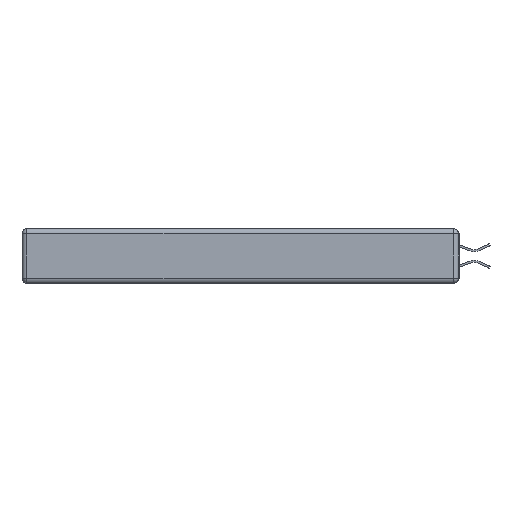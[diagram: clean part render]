
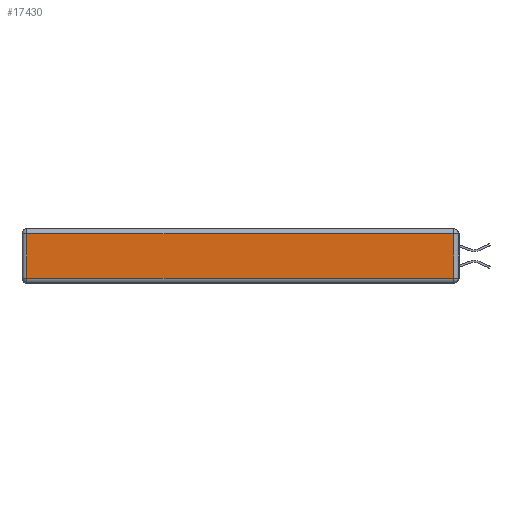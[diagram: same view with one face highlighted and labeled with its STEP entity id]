
A CAD part, left-side view. The second image highlights one B-rep face of the part: STEP entity #17430.
In plain terms, the highlighted planar face has unit normal (-1, 0, 0).
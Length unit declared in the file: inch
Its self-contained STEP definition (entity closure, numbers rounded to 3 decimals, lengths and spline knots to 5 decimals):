
#206 = ORIENTED_EDGE ( 'NONE', *, *, #7470, .T. ) ;
#953 = ORIENTED_EDGE ( 'NONE', *, *, #4564, .T. ) ;
#1438 = LINE ( 'NONE', #15398, #14911 ) ;
#2164 = VECTOR ( 'NONE', #7937, 39.37008 ) ;
#2230 = CARTESIAN_POINT ( 'NONE',  ( 0., 2.75, -0.03 ) ) ;
#3744 = VERTEX_POINT ( 'NONE', #12139 ) ;
#4537 = DIRECTION ( 'NONE',  ( 0., -1., 0. ) ) ;
#4564 = EDGE_CURVE ( 'NONE', #11316, #7080, #1438, .T. ) ;
#4608 = CARTESIAN_POINT ( 'NONE',  ( 0., 0.03, -0.343 ) ) ;
#4664 = DIRECTION ( 'NONE',  ( -1., 0., 0. ) ) ;
#5738 = EDGE_LOOP ( 'NONE', ( #206, #11890, #14962, #953 ) ) ;
#5791 = LINE ( 'NONE', #4608, #2164 ) ;
#6066 = CARTESIAN_POINT ( 'NONE',  ( 0., 0.03, -0.313 ) ) ;
#7080 = VERTEX_POINT ( 'NONE', #13982 ) ;
#7470 = EDGE_CURVE ( 'NONE', #7080, #8627, #12040, .T. ) ;
#7937 = DIRECTION ( 'NONE',  ( 0., 0., 1. ) ) ;
#8220 = VECTOR ( 'NONE', #4537, 39.37008 ) ;
#8518 = VECTOR ( 'NONE', #10351, 39.37008 ) ;
#8627 = VERTEX_POINT ( 'NONE', #6066 ) ;
#8651 = DIRECTION ( 'NONE',  ( 0., 0., -1. ) ) ;
#10269 = CARTESIAN_POINT ( 'NONE',  ( 0., 0., -0.343 ) ) ;
#10351 = DIRECTION ( 'NONE',  ( 0., 1., 0. ) ) ;
#11195 = EDGE_CURVE ( 'NONE', #3744, #11316, #17252, .T. ) ;
#11316 = VERTEX_POINT ( 'NONE', #12196 ) ;
#11890 = ORIENTED_EDGE ( 'NONE', *, *, #17446, .T. ) ;
#12040 = LINE ( 'NONE', #13924, #8220 ) ;
#12139 = CARTESIAN_POINT ( 'NONE',  ( 0., 0.03, -0.03 ) ) ;
#12196 = CARTESIAN_POINT ( 'NONE',  ( 0., 2.72, -0.03 ) ) ;
#12855 = PLANE ( 'NONE',  #13074 ) ;
#13074 = AXIS2_PLACEMENT_3D ( 'NONE', #10269, #4664, #14212 ) ;
#13075 = FACE_OUTER_BOUND ( 'NONE', #5738, .T. ) ;
#13924 = CARTESIAN_POINT ( 'NONE',  ( 0., 0., -0.313 ) ) ;
#13982 = CARTESIAN_POINT ( 'NONE',  ( 0., 2.72, -0.313 ) ) ;
#14212 = DIRECTION ( 'NONE',  ( 0., 0., 1. ) ) ;
#14911 = VECTOR ( 'NONE', #8651, 39.37008 ) ;
#14962 = ORIENTED_EDGE ( 'NONE', *, *, #11195, .T. ) ;
#15398 = CARTESIAN_POINT ( 'NONE',  ( 0., 2.72, -0.343 ) ) ;
#17252 = LINE ( 'NONE', #2230, #8518 ) ;
#17430 = ADVANCED_FACE ( 'NONE', ( #13075 ), #12855, .T. ) ;
#17446 = EDGE_CURVE ( 'NONE', #8627, #3744, #5791, .T. ) ;
